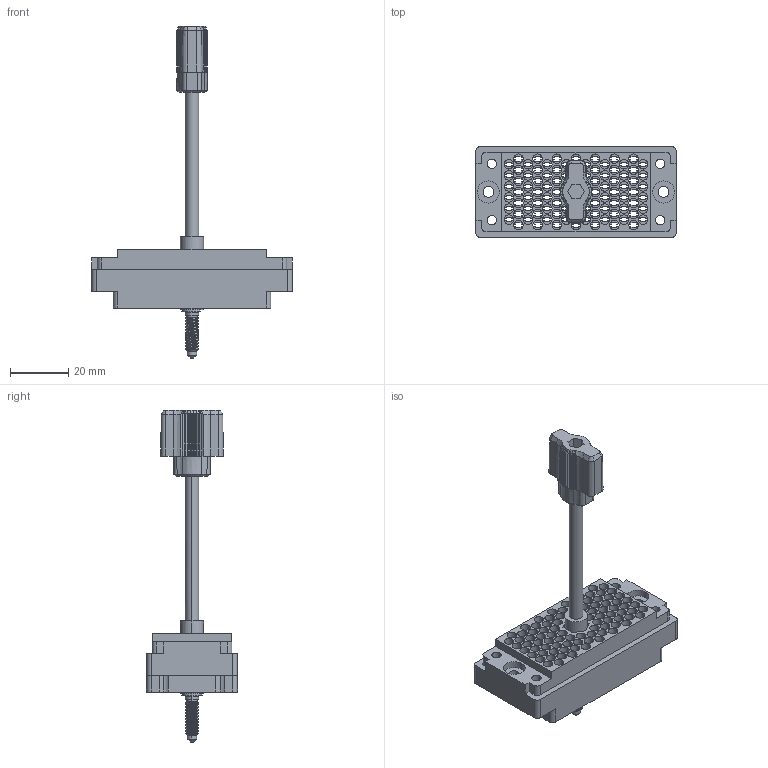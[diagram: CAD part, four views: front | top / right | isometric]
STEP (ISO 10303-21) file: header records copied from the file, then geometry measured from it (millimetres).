
FILE_DESCRIPTION (( 'STEP AP203' ), '1' );
FILE_NAME ('516-090-000-105.STEP', '2020-03-10T15:25:46', ( '' ), ( '' ), 'SwSTEP 2.0', 'SolidWorks 2016', '' );
FILE_SCHEMA (( 'CONFIG_CONTROL_DESIGN' ));
Length unit declared in the file: inch
Products named in the file (9): 516-251-095-100; 516-253-190-107; 516 Plug Insulator_090; 516-253-095-100; 516-254-091-109; 516-090-000-105; 516-250-091-111; Actuating Screw Assy 090-120; Grub Screw
Assembly tree (9 placements, depth 3):
  516-090-000-105
    516 Plug Insulator_090
    Actuating Screw Assy 090-120
      516-251-095-100
      516-254-091-109
      516-253-095-100  x2
      516-253-190-107
      516-250-091-111
      Grub Screw
Bounding box: 69.04 x 31.34 x 114.34 mm (x, y, z)
Volume: 21713.9 mm3; surface area: 26576 mm2
Topology: 8 solids, 8 shells, 2149 faces, 6255 edges, 4142 vertices
Faces by surface type: plane 1495, cylinder 575, cone 62, bspline 17
Entity records: 78846 total; most frequent: CARTESIAN_POINT 19823, ORIENTED_EDGE 12486, DIRECTION 11837, EDGE_CURVE 6243, VECTOR 4533, LINE 4533, VERTEX_POINT 4134, AXIS2_PLACEMENT_3D 3652
